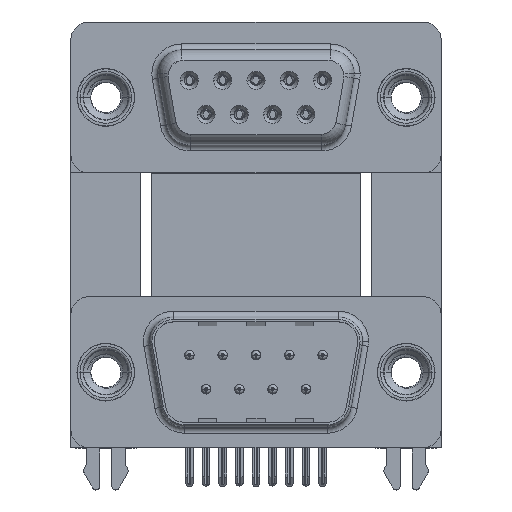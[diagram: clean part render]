
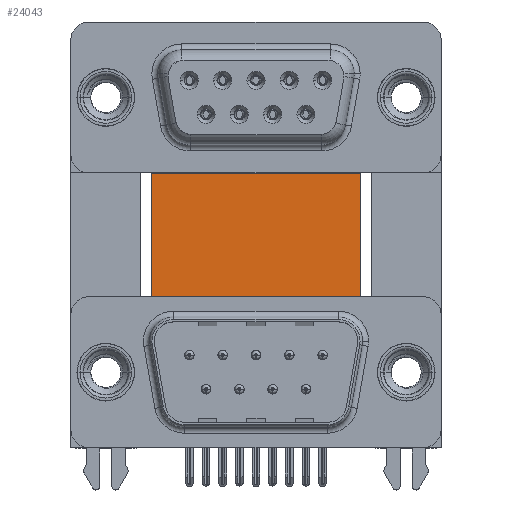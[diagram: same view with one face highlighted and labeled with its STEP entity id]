
A CAD part, top view. The second image highlights one B-rep face of the part: STEP entity #24043.
In plain terms, the highlighted planar face has unit normal (0, 0, 1).
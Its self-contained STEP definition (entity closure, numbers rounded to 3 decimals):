
#121 = LINE ( 'NONE', #24476, #31390 ) ;
#221 = ORIENTED_EDGE ( 'NONE', *, *, #3547, .T. ) ;
#1466 = PLANE ( 'NONE',  #14629 ) ;
#2137 = LINE ( 'NONE', #17197, #22489 ) ;
#2264 = VECTOR ( 'NONE', #16004, 1000. ) ;
#3082 = ORIENTED_EDGE ( 'NONE', *, *, #4477, .T. ) ;
#3547 = EDGE_CURVE ( 'NONE', #14159, #8437, #2137, .T. ) ;
#3915 = ORIENTED_EDGE ( 'NONE', *, *, #15781, .T. ) ;
#4055 = VERTEX_POINT ( 'NONE', #9353 ) ;
#4318 = VERTEX_POINT ( 'NONE', #34077 ) ;
#4449 = CARTESIAN_POINT ( 'NONE',  ( 3.79, 16.585, -12. ) ) ;
#4477 = EDGE_CURVE ( 'NONE', #4055, #8195, #27372, .T. ) ;
#4625 = CARTESIAN_POINT ( 'NONE',  ( 3.79, 16.585, -12. ) ) ;
#6050 = VERTEX_POINT ( 'NONE', #11299 ) ;
#6158 = VECTOR ( 'NONE', #29581, 1000. ) ;
#6309 = VECTOR ( 'NONE', #18869, 1000. ) ;
#6630 = ORIENTED_EDGE ( 'NONE', *, *, #29398, .T. ) ;
#7509 = CARTESIAN_POINT ( 'NONE',  ( 21.2, -0.735, -12. ) ) ;
#8195 = VERTEX_POINT ( 'NONE', #31069 ) ;
#8437 = VERTEX_POINT ( 'NONE', #34352 ) ;
#8514 = ORIENTED_EDGE ( 'NONE', *, *, #25885, .T. ) ;
#9135 = LINE ( 'NONE', #33541, #30093 ) ;
#9353 = CARTESIAN_POINT ( 'NONE',  ( 22.09, -4.635, -12. ) ) ;
#10098 = EDGE_CURVE ( 'NONE', #15838, #30442, #26059, .T. ) ;
#10432 = EDGE_CURVE ( 'NONE', #15838, #6050, #19861, .T. ) ;
#11299 = CARTESIAN_POINT ( 'NONE',  ( 21.2, 16.585, -12. ) ) ;
#11658 = ORIENTED_EDGE ( 'NONE', *, *, #10098, .T. ) ;
#12319 = DIRECTION ( 'NONE',  ( 0., -1., 0. ) ) ;
#12510 = DIRECTION ( 'NONE',  ( 0., -1., 0. ) ) ;
#12583 = DIRECTION ( 'NONE',  ( -0.336, -0.942, 0. ) ) ;
#12879 = CARTESIAN_POINT ( 'NONE',  ( 3.79, -3.735, -12. ) ) ;
#14159 = VERTEX_POINT ( 'NONE', #32817 ) ;
#14629 = AXIS2_PLACEMENT_3D ( 'NONE', #4449, #19289, #34177 ) ;
#15781 = EDGE_CURVE ( 'NONE', #4318, #4055, #29798, .T. ) ;
#15838 = VERTEX_POINT ( 'NONE', #24021 ) ;
#16004 = DIRECTION ( 'NONE',  ( 0., -1., 0. ) ) ;
#16902 = FACE_OUTER_BOUND ( 'NONE', #21825, .T. ) ;
#17197 = CARTESIAN_POINT ( 'NONE',  ( 2.9, -4.635, -12. ) ) ;
#17266 = ORIENTED_EDGE ( 'NONE', *, *, #36795, .F. ) ;
#17441 = VECTOR ( 'NONE', #28607, 1000. ) ;
#18869 = DIRECTION ( 'NONE',  ( 1., 0., 0. ) ) ;
#18950 = VECTOR ( 'NONE', #23592, 1000. ) ;
#19289 = DIRECTION ( 'NONE',  ( 0., 0., -1. ) ) ;
#19806 = LINE ( 'NONE', #25958, #30085 ) ;
#19861 = LINE ( 'NONE', #4625, #17441 ) ;
#21030 = CARTESIAN_POINT ( 'NONE',  ( 22.09, -4.635, -12. ) ) ;
#21825 = EDGE_LOOP ( 'NONE', ( #39032, #3915, #3082, #34651, #17266, #27960, #11658, #6630, #221, #8514 ) ) ;
#22021 = LINE ( 'NONE', #12879, #6309 ) ;
#22489 = VECTOR ( 'NONE', #30009, 1000. ) ;
#23592 = DIRECTION ( 'NONE',  ( -0.336, 0.942, 0. ) ) ;
#24021 = CARTESIAN_POINT ( 'NONE',  ( 3.79, 16.585, -12. ) ) ;
#24043 = ADVANCED_FACE ( 'NONE', ( #16902 ), #1466, .F. ) ;
#24476 = CARTESIAN_POINT ( 'NONE',  ( 2.4, -4.635, -12. ) ) ;
#25885 = EDGE_CURVE ( 'NONE', #8437, #28805, #19806, .T. ) ;
#25958 = CARTESIAN_POINT ( 'NONE',  ( 2.9, -3.735, -12. ) ) ;
#26059 = LINE ( 'NONE', #38143, #2264 ) ;
#26590 = CARTESIAN_POINT ( 'NONE',  ( 22.59, -4.635, -12. ) ) ;
#27372 = LINE ( 'NONE', #21030, #6158 ) ;
#27384 = VERTEX_POINT ( 'NONE', #7509 ) ;
#27960 = ORIENTED_EDGE ( 'NONE', *, *, #10432, .F. ) ;
#28607 = DIRECTION ( 'NONE',  ( 1., 0., 0. ) ) ;
#28805 = VERTEX_POINT ( 'NONE', #33655 ) ;
#29398 = EDGE_CURVE ( 'NONE', #30442, #14159, #121, .T. ) ;
#29581 = DIRECTION ( 'NONE',  ( 1., 0., 0. ) ) ;
#29584 = LINE ( 'NONE', #26590, #18950 ) ;
#29798 = LINE ( 'NONE', #30386, #33943 ) ;
#30009 = DIRECTION ( 'NONE',  ( 1., 0., 0. ) ) ;
#30085 = VECTOR ( 'NONE', #38431, 1000. ) ;
#30093 = VECTOR ( 'NONE', #12510, 1000. ) ;
#30386 = CARTESIAN_POINT ( 'NONE',  ( 22.09, -3.735, -12. ) ) ;
#30442 = VERTEX_POINT ( 'NONE', #34901 ) ;
#31069 = CARTESIAN_POINT ( 'NONE',  ( 22.59, -4.635, -12. ) ) ;
#31390 = VECTOR ( 'NONE', #12583, 1000. ) ;
#32817 = CARTESIAN_POINT ( 'NONE',  ( 2.4, -4.635, -12. ) ) ;
#33541 = CARTESIAN_POINT ( 'NONE',  ( 21.2, 16.585, -12. ) ) ;
#33655 = CARTESIAN_POINT ( 'NONE',  ( 2.9, -3.735, -12. ) ) ;
#33943 = VECTOR ( 'NONE', #12319, 1000. ) ;
#34077 = CARTESIAN_POINT ( 'NONE',  ( 22.09, -3.735, -12. ) ) ;
#34177 = DIRECTION ( 'NONE',  ( -1., 0., 0. ) ) ;
#34352 = CARTESIAN_POINT ( 'NONE',  ( 2.9, -4.635, -12. ) ) ;
#34651 = ORIENTED_EDGE ( 'NONE', *, *, #35479, .T. ) ;
#34901 = CARTESIAN_POINT ( 'NONE',  ( 3.79, -0.735, -12. ) ) ;
#35479 = EDGE_CURVE ( 'NONE', #8195, #27384, #29584, .T. ) ;
#35707 = EDGE_CURVE ( 'NONE', #28805, #4318, #22021, .T. ) ;
#36795 = EDGE_CURVE ( 'NONE', #6050, #27384, #9135, .T. ) ;
#38143 = CARTESIAN_POINT ( 'NONE',  ( 3.79, 16.585, -12. ) ) ;
#38431 = DIRECTION ( 'NONE',  ( 0., 1., 0. ) ) ;
#39032 = ORIENTED_EDGE ( 'NONE', *, *, #35707, .T. ) ;
